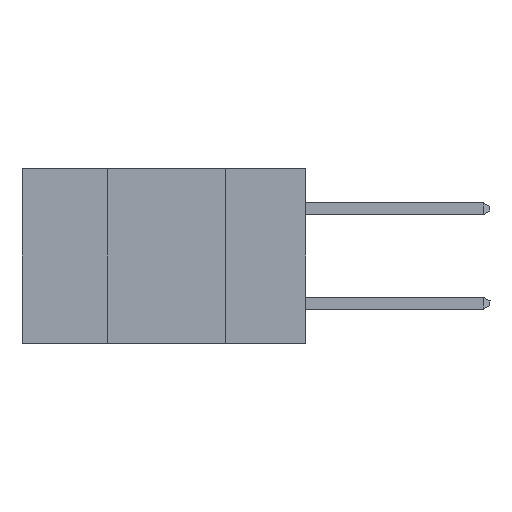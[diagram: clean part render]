
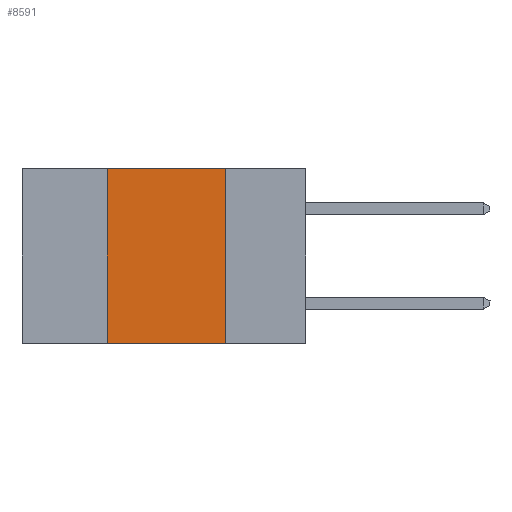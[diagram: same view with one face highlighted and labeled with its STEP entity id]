
A CAD part, left-side view. The second image highlights one B-rep face of the part: STEP entity #8591.
In plain terms, the highlighted planar face has unit normal (-1, 0, 0).
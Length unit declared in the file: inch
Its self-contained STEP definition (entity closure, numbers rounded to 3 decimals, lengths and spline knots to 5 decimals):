
#92 = ORIENTED_EDGE ( 'NONE', *, *, #3055, .F. ) ;
#424 = CARTESIAN_POINT ( 'NONE',  ( 0., 0.6, 0. ) ) ;
#900 = CARTESIAN_POINT ( 'NONE',  ( 0., 0.6, 0. ) ) ;
#1254 = LINE ( 'NONE', #10081, #15886 ) ;
#2289 = EDGE_CURVE ( 'NONE', #5214, #7778, #17454, .T. ) ;
#2437 = CARTESIAN_POINT ( 'NONE',  ( 0., 0.17, 0. ) ) ;
#3055 = EDGE_CURVE ( 'NONE', #5263, #5214, #9171, .T. ) ;
#3851 = CARTESIAN_POINT ( 'NONE',  ( 0., 0.6, -0.37 ) ) ;
#4236 = DIRECTION ( 'NONE',  ( 0., 0., -1. ) ) ;
#4594 = FACE_OUTER_BOUND ( 'NONE', #19117, .T. ) ;
#4958 = AXIS2_PLACEMENT_3D ( 'NONE', #424, #8502, #21064 ) ;
#5214 = VERTEX_POINT ( 'NONE', #7092 ) ;
#5263 = VERTEX_POINT ( 'NONE', #9128 ) ;
#5531 = EDGE_CURVE ( 'NONE', #7778, #11189, #1254, .T. ) ;
#5827 = EDGE_CURVE ( 'NONE', #5263, #11189, #13319, .T. ) ;
#7092 = CARTESIAN_POINT ( 'NONE',  ( 0., 0.42, 0. ) ) ;
#7778 = VERTEX_POINT ( 'NONE', #2437 ) ;
#8502 = DIRECTION ( 'NONE',  ( 1., 0., 0. ) ) ;
#8591 = ADVANCED_FACE ( 'NONE', ( #4594 ), #17574, .F. ) ;
#8846 = ORIENTED_EDGE ( 'NONE', *, *, #5531, .F. ) ;
#9128 = CARTESIAN_POINT ( 'NONE',  ( 0., 0.42, -0.37 ) ) ;
#9171 = LINE ( 'NONE', #12034, #22867 ) ;
#10081 = CARTESIAN_POINT ( 'NONE',  ( 0., 0.17, -0.37 ) ) ;
#11189 = VERTEX_POINT ( 'NONE', #12701 ) ;
#11977 = DIRECTION ( 'NONE',  ( 0., 0., 1. ) ) ;
#12034 = CARTESIAN_POINT ( 'NONE',  ( 0., 0.42, -0.37 ) ) ;
#12669 = VECTOR ( 'NONE', #18997, 39.37008 ) ;
#12701 = CARTESIAN_POINT ( 'NONE',  ( 0., 0.17, -0.37 ) ) ;
#13319 = LINE ( 'NONE', #3851, #22166 ) ;
#14840 = ORIENTED_EDGE ( 'NONE', *, *, #2289, .F. ) ;
#15137 = DIRECTION ( 'NONE',  ( 0., -1., 0. ) ) ;
#15886 = VECTOR ( 'NONE', #4236, 39.37008 ) ;
#17454 = LINE ( 'NONE', #900, #12669 ) ;
#17574 = PLANE ( 'NONE',  #4958 ) ;
#17704 = ORIENTED_EDGE ( 'NONE', *, *, #5827, .T. ) ;
#18997 = DIRECTION ( 'NONE',  ( 0., -1., 0. ) ) ;
#19117 = EDGE_LOOP ( 'NONE', ( #8846, #14840, #92, #17704 ) ) ;
#21064 = DIRECTION ( 'NONE',  ( 0., 0., -1. ) ) ;
#22166 = VECTOR ( 'NONE', #15137, 39.37008 ) ;
#22867 = VECTOR ( 'NONE', #11977, 39.37008 ) ;
